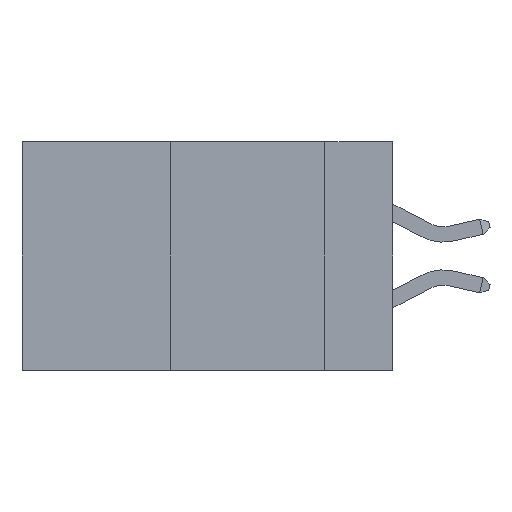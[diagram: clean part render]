
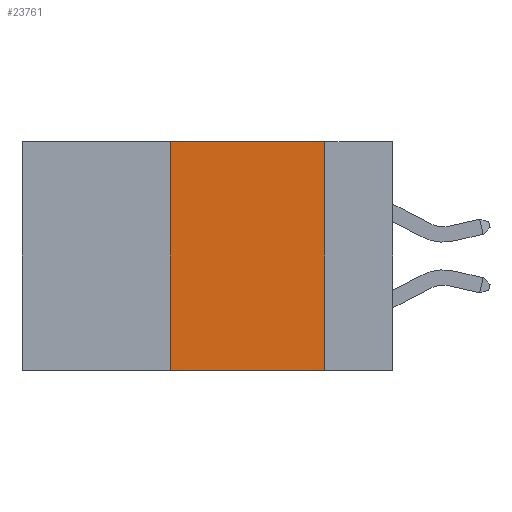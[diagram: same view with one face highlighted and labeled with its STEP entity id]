
A CAD part, left-side view. The second image highlights one B-rep face of the part: STEP entity #23761.
In plain terms, the highlighted planar face has unit normal (-1, 0, 0).
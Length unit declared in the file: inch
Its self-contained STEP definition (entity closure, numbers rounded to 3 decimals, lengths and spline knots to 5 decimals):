
#443 = DIRECTION ( 'NONE',  ( 0., 0., -1. ) ) ;
#752 = VECTOR ( 'NONE', #14076, 39.37008 ) ;
#1049 = EDGE_LOOP ( 'NONE', ( #15456, #20032, #17983, #30082 ) ) ;
#1160 = EDGE_CURVE ( 'NONE', #29314, #4849, #15752, .T. ) ;
#2098 = VECTOR ( 'NONE', #19524, 39.37008 ) ;
#2444 = LINE ( 'NONE', #24693, #752 ) ;
#3271 = CARTESIAN_POINT ( 'NONE',  ( 0., 0.6, 0. ) ) ;
#4849 = VERTEX_POINT ( 'NONE', #19120 ) ;
#6256 = DIRECTION ( 'NONE',  ( 1., 0., 0. ) ) ;
#7241 = VERTEX_POINT ( 'NONE', #13358 ) ;
#7710 = DIRECTION ( 'NONE',  ( 0., 0., -1. ) ) ;
#12109 = EDGE_CURVE ( 'NONE', #7241, #14051, #29882, .T. ) ;
#12789 = CARTESIAN_POINT ( 'NONE',  ( 0., 0.36, -0.37 ) ) ;
#13121 = CARTESIAN_POINT ( 'NONE',  ( 0., 0.11, -0.37 ) ) ;
#13236 = CARTESIAN_POINT ( 'NONE',  ( 0., 0.11, 0. ) ) ;
#13358 = CARTESIAN_POINT ( 'NONE',  ( 0., 0.11, 0. ) ) ;
#14051 = VERTEX_POINT ( 'NONE', #13121 ) ;
#14076 = DIRECTION ( 'NONE',  ( 0., -1., 0. ) ) ;
#15456 = ORIENTED_EDGE ( 'NONE', *, *, #12109, .F. ) ;
#15752 = LINE ( 'NONE', #30369, #2098 ) ;
#17332 = DIRECTION ( 'NONE',  ( 0., -1., 0. ) ) ;
#17983 = ORIENTED_EDGE ( 'NONE', *, *, #1160, .F. ) ;
#18798 = VECTOR ( 'NONE', #7710, 39.37008 ) ;
#19120 = CARTESIAN_POINT ( 'NONE',  ( 0., 0.36, 0. ) ) ;
#19524 = DIRECTION ( 'NONE',  ( 0., 0., 1. ) ) ;
#20032 = ORIENTED_EDGE ( 'NONE', *, *, #31008, .F. ) ;
#22256 = PLANE ( 'NONE',  #25780 ) ;
#22695 = CARTESIAN_POINT ( 'NONE',  ( 0., 0.6, 0. ) ) ;
#23165 = EDGE_CURVE ( 'NONE', #29314, #14051, #2444, .T. ) ;
#23761 = ADVANCED_FACE ( 'NONE', ( #32694 ), #22256, .F. ) ;
#24693 = CARTESIAN_POINT ( 'NONE',  ( 0., 0.6, -0.37 ) ) ;
#25780 = AXIS2_PLACEMENT_3D ( 'NONE', #3271, #6256, #443 ) ;
#29314 = VERTEX_POINT ( 'NONE', #12789 ) ;
#29882 = LINE ( 'NONE', #13236, #18798 ) ;
#30082 = ORIENTED_EDGE ( 'NONE', *, *, #23165, .T. ) ;
#30207 = LINE ( 'NONE', #22695, #34438 ) ;
#30369 = CARTESIAN_POINT ( 'NONE',  ( 0., 0.36, 0. ) ) ;
#31008 = EDGE_CURVE ( 'NONE', #4849, #7241, #30207, .T. ) ;
#32694 = FACE_OUTER_BOUND ( 'NONE', #1049, .T. ) ;
#34438 = VECTOR ( 'NONE', #17332, 39.37008 ) ;
